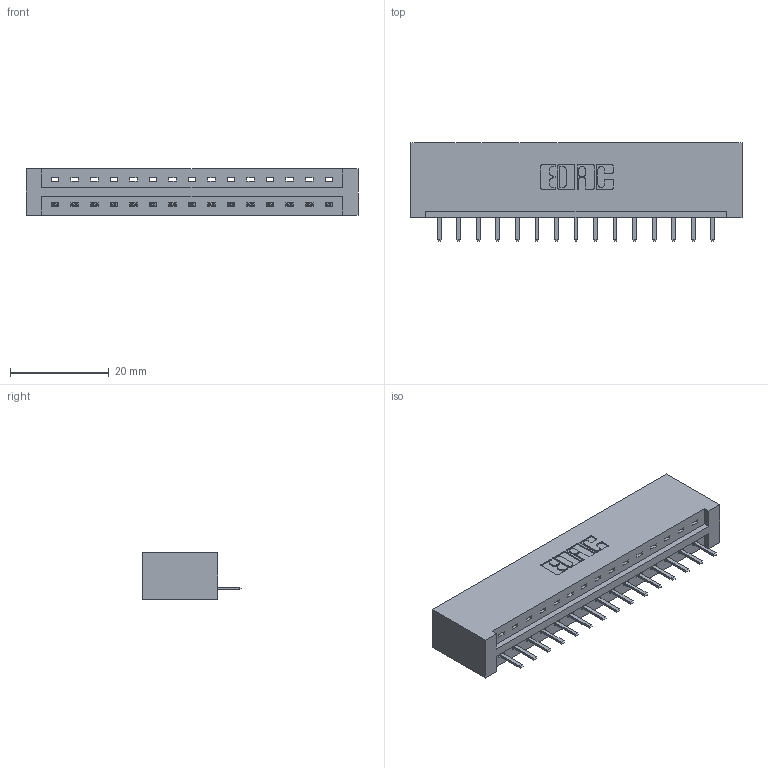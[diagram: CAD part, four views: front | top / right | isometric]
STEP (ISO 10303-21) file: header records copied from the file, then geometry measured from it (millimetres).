
FILE_DESCRIPTION (( 'STEP AP203' ), '1' );
FILE_NAME ('387-015-520-101.STEP', '2019-10-02T16:11:27', ( '' ), ( '' ), 'SwSTEP 2.0', 'SolidWorks 2016', '' );
FILE_SCHEMA (( 'CONFIG_CONTROL_DESIGN' ));
Length unit declared in the file: inch
Products named in the file (3): 337 Part_No Mounting Lugs; 387-015-520-101; 345-292-001_345-293-120
Assembly tree (16 placements, depth 2):
  387-015-520-101
    337 Part_No Mounting Lugs
    345-292-001_345-293-120  x15
Bounding box: 67.31 x 20.02 x 9.4 mm (x, y, z)
Volume: 7353.4 mm3; surface area: 7275 mm2
Topology: 16 solids, 16 shells, 1096 faces, 3227 edges, 2110 vertices
Faces by surface type: plane 786, cylinder 310
Entity records: 14479 total; most frequent: CARTESIAN_POINT 2539, ORIENTED_EDGE 2478, DIRECTION 2173, EDGE_CURVE 1239, VECTOR 1115, LINE 1115, VERTEX_POINT 822, AXIS2_PLACEMENT_3D 529
